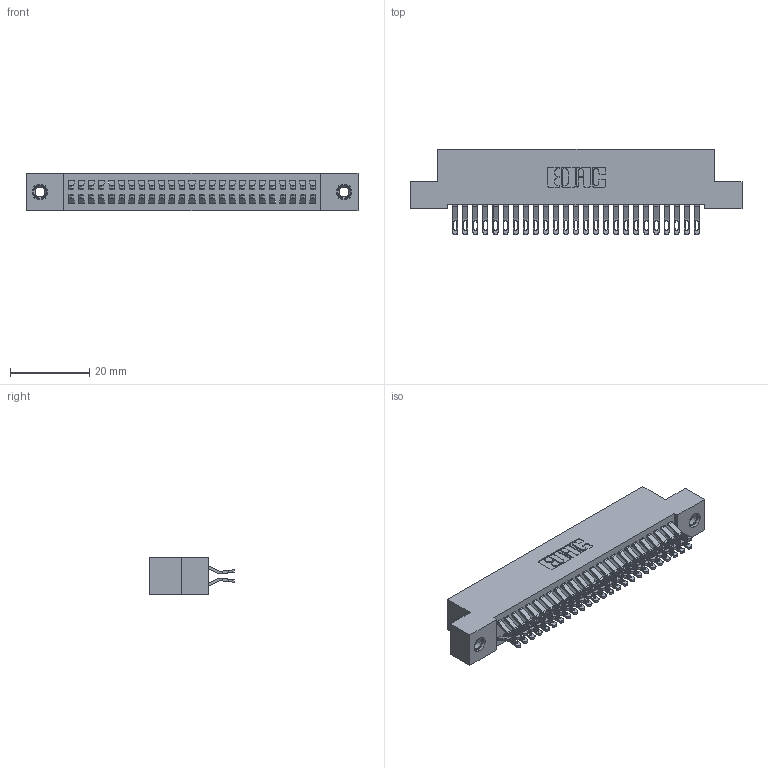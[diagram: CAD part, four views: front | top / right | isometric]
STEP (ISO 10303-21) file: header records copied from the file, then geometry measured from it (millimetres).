
FILE_DESCRIPTION (( 'STEP AP203' ), '1' );
FILE_NAME ('392-050-555-207.STEP', '2019-10-08T11:35:54', ( '' ), ( '' ), 'SwSTEP 2.0', 'SolidWorks 2016', '' );
FILE_SCHEMA (( 'CONFIG_CONTROL_DESIGN' ));
Length unit declared in the file: inch
Products named in the file (4): 392-050-555-207; 342 Part_TI; 345-292-001_555 Tail; 345-250-001_345-250-005-103
Assembly tree (53 placements, depth 2):
  392-050-555-207
    342 Part_TI
    345-292-001_555 Tail  x50
    345-250-001_345-250-005-103  x2
Bounding box: 83.82 x 21.47 x 9.4 mm (x, y, z)
Volume: 7577 mm3; surface area: 12424.1 mm2
Topology: 53 solids, 53 shells, 3070 faces, 9585 edges, 6382 vertices
Faces by surface type: plane 1798, cylinder 1256, cone 12, torus 4
Entity records: 19662 total; most frequent: CARTESIAN_POINT 3295, ORIENTED_EDGE 3194, DIRECTION 2847, EDGE_CURVE 1597, VECTOR 1429, LINE 1429, VERTEX_POINT 1060, AXIS2_PLACEMENT_3D 709
